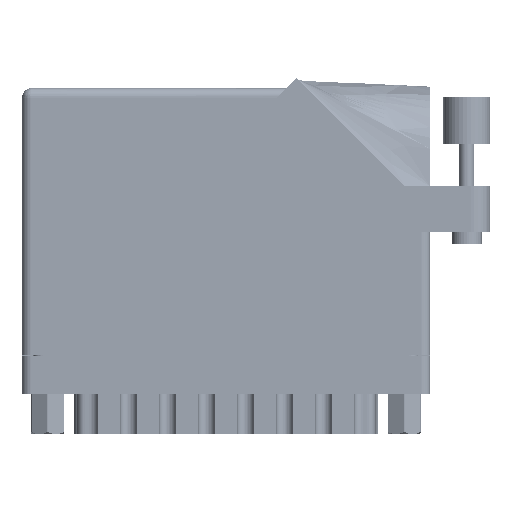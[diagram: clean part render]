
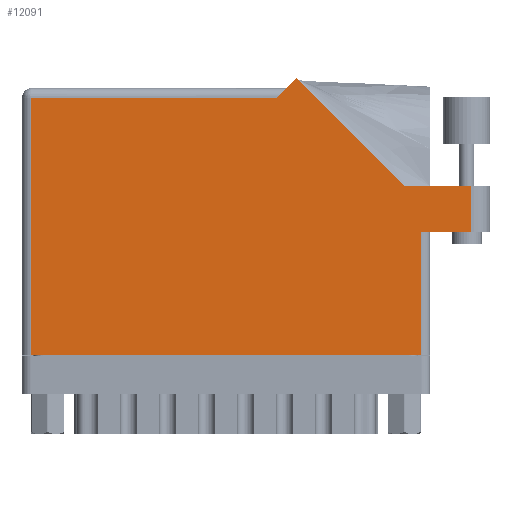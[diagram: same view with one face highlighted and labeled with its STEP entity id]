
A CAD part, front view. The second image highlights one B-rep face of the part: STEP entity #12091.
In plain terms, the highlighted face is planar.
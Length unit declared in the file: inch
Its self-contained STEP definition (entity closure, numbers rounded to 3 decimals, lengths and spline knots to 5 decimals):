
#484 = CARTESIAN_POINT ( 'NONE',  ( 0., 0., 0. ) ) ;
#1533 = VERTEX_POINT ( 'NONE', #51182 ) ;
#3441 = DIRECTION ( 'NONE',  ( 0., 0., -1. ) ) ;
#4492 = ORIENTED_EDGE ( 'NONE', *, *, #73438, .T. ) ;
#6046 = CARTESIAN_POINT ( 'NONE',  ( 0., 1.713, 0. ) ) ;
#6386 = ORIENTED_EDGE ( 'NONE', *, *, #54478, .T. ) ;
#7234 = ORIENTED_EDGE ( 'NONE', *, *, #59462, .T. ) ;
#9529 = CARTESIAN_POINT ( 'NONE',  ( 2.656, 0.815, 0. ) ) ;
#9607 = EDGE_LOOP ( 'NONE', ( #72598, #85807, #37431, #45136, #77863, #53129, #6386, #4492, #7234 ) ) ;
#9914 = VERTEX_POINT ( 'NONE', #43702 ) ;
#10028 = CARTESIAN_POINT ( 'NONE',  ( 2.993, 1.122, 0. ) ) ;
#10420 = DIRECTION ( 'NONE',  ( -1., 0., 0. ) ) ;
#10753 = CARTESIAN_POINT ( 'NONE',  ( 1.696, 1.713, 0. ) ) ;
#12091 = ADVANCED_FACE ( 'NONE', ( #76202 ), #70511, .F. ) ;
#13036 = DIRECTION ( 'NONE',  ( -1., 0., 0. ) ) ;
#13168 = VERTEX_POINT ( 'NONE', #72034 ) ;
#14058 = VECTOR ( 'NONE', #82671, 39.37008 ) ;
#15343 = VECTOR ( 'NONE', #29215, 39.37008 ) ;
#16219 = EDGE_CURVE ( 'NONE', #38372, #9914, #55965, .T. ) ;
#16718 = DIRECTION ( 'NONE',  ( 0., -1., 0. ) ) ;
#17032 = CARTESIAN_POINT ( 'NONE',  ( 2.656, 0.815, 0. ) ) ;
#21400 = CARTESIAN_POINT ( 'NONE',  ( 2.656, 0., 0. ) ) ;
#21470 = VECTOR ( 'NONE', #81067, 39.37008 ) ;
#24016 = DIRECTION ( 'NONE',  ( 0., 1., 0. ) ) ;
#24122 = VECTOR ( 'NONE', #24016, 39.37008 ) ;
#24127 = EDGE_CURVE ( 'NONE', #45270, #24704, #54064, .T. ) ;
#24704 = VERTEX_POINT ( 'NONE', #10753 ) ;
#25300 = EDGE_CURVE ( 'NONE', #24704, #13168, #39178, .T. ) ;
#26228 = EDGE_CURVE ( 'NONE', #9914, #1533, #69268, .T. ) ;
#27068 = CARTESIAN_POINT ( 'NONE',  ( 1.758, 1.775, 0. ) ) ;
#28625 = CARTESIAN_POINT ( 'NONE',  ( 1.82871, 1.84571, 0. ) ) ;
#29058 = VECTOR ( 'NONE', #69459, 39.37008 ) ;
#29215 = DIRECTION ( 'NONE',  ( 0., 1., 0. ) ) ;
#30210 = LINE ( 'NONE', #76813, #59843 ) ;
#30334 = VECTOR ( 'NONE', #34023, 39.37008 ) ;
#30874 = EDGE_CURVE ( 'NONE', #1533, #80407, #72706, .T. ) ;
#34023 = DIRECTION ( 'NONE',  ( -0.707, -0.707, 0. ) ) ;
#36658 = LINE ( 'NONE', #48904, #43523 ) ;
#37431 = ORIENTED_EDGE ( 'NONE', *, *, #30874, .T. ) ;
#38354 = LINE ( 'NONE', #17032, #24122 ) ;
#38372 = VERTEX_POINT ( 'NONE', #9529 ) ;
#39178 = LINE ( 'NONE', #6046, #14058 ) ;
#42684 = CARTESIAN_POINT ( 'NONE',  ( 2.55242, 1.122, 0. ) ) ;
#42773 = DIRECTION ( 'NONE',  ( -0.707, 0.707, 0. ) ) ;
#43523 = VECTOR ( 'NONE', #42773, 39.37008 ) ;
#43702 = CARTESIAN_POINT ( 'NONE',  ( 2.993, 0.815, 0. ) ) ;
#45136 = ORIENTED_EDGE ( 'NONE', *, *, #71602, .T. ) ;
#45268 = CARTESIAN_POINT ( 'NONE',  ( 3.118, 1.122, 0. ) ) ;
#45270 = VERTEX_POINT ( 'NONE', #28625 ) ;
#47122 = LINE ( 'NONE', #484, #21470 ) ;
#48904 = CARTESIAN_POINT ( 'NONE',  ( 2.55242, 1.122, 0. ) ) ;
#51182 = CARTESIAN_POINT ( 'NONE',  ( 2.993, 1.122, 0. ) ) ;
#53129 = ORIENTED_EDGE ( 'NONE', *, *, #25300, .T. ) ;
#54064 = LINE ( 'NONE', #27068, #30334 ) ;
#54478 = EDGE_CURVE ( 'NONE', #13168, #56040, #30210, .T. ) ;
#55965 = LINE ( 'NONE', #75148, #29058 ) ;
#56040 = VERTEX_POINT ( 'NONE', #72950 ) ;
#59462 = EDGE_CURVE ( 'NONE', #64435, #38372, #38354, .T. ) ;
#59843 = VECTOR ( 'NONE', #16718, 39.37008 ) ;
#64435 = VERTEX_POINT ( 'NONE', #21400 ) ;
#69268 = LINE ( 'NONE', #10028, #15343 ) ;
#69459 = DIRECTION ( 'NONE',  ( 1., 0., 0. ) ) ;
#70511 = PLANE ( 'NONE',  #79464 ) ;
#71602 = EDGE_CURVE ( 'NONE', #80407, #45270, #36658, .T. ) ;
#72034 = CARTESIAN_POINT ( 'NONE',  ( 0.062, 1.713, 0. ) ) ;
#72598 = ORIENTED_EDGE ( 'NONE', *, *, #16219, .T. ) ;
#72706 = LINE ( 'NONE', #45268, #80907 ) ;
#72950 = CARTESIAN_POINT ( 'NONE',  ( 0.062, 0., 0. ) ) ;
#73438 = EDGE_CURVE ( 'NONE', #56040, #64435, #47122, .T. ) ;
#75148 = CARTESIAN_POINT ( 'NONE',  ( 2.718, 0.815, 0. ) ) ;
#75788 = CARTESIAN_POINT ( 'NONE',  ( 0., 1.775, 0. ) ) ;
#76202 = FACE_OUTER_BOUND ( 'NONE', #9607, .T. ) ;
#76813 = CARTESIAN_POINT ( 'NONE',  ( 0.062, 0., 0. ) ) ;
#77863 = ORIENTED_EDGE ( 'NONE', *, *, #24127, .T. ) ;
#79464 = AXIS2_PLACEMENT_3D ( 'NONE', #75788, #3441, #10420 ) ;
#80407 = VERTEX_POINT ( 'NONE', #42684 ) ;
#80907 = VECTOR ( 'NONE', #13036, 39.37008 ) ;
#81067 = DIRECTION ( 'NONE',  ( 1., 0., 0. ) ) ;
#82671 = DIRECTION ( 'NONE',  ( -1., 0., 0. ) ) ;
#85807 = ORIENTED_EDGE ( 'NONE', *, *, #26228, .T. ) ;
